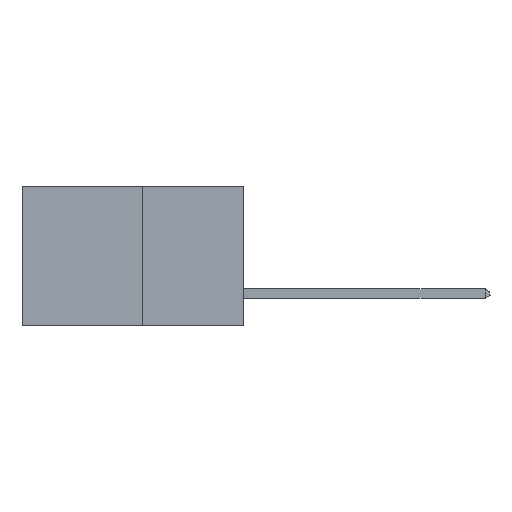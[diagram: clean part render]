
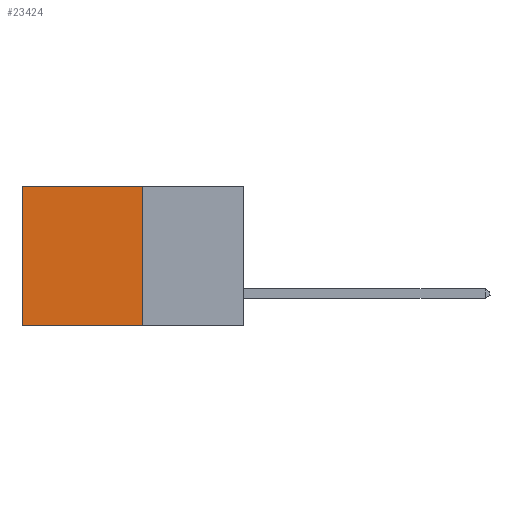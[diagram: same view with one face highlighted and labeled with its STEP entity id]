
A CAD part, left-side view. The second image highlights one B-rep face of the part: STEP entity #23424.
In plain terms, the highlighted planar face has unit normal (-1, 0, 0).
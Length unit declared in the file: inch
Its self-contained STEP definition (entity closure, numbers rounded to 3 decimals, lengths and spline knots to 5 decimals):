
#1479 = CARTESIAN_POINT ( 'NONE',  ( 0.277, 0.59, -0.37 ) ) ;
#3190 = CARTESIAN_POINT ( 'NONE',  ( 0.277, 0.27, -0.37 ) ) ;
#3373 = EDGE_LOOP ( 'NONE', ( #11371, #21034, #13658, #12511 ) ) ;
#3605 = DIRECTION ( 'NONE',  ( 0., 0., -1. ) ) ;
#3634 = CARTESIAN_POINT ( 'NONE',  ( 0.277, 0.27, -0.37 ) ) ;
#5493 = CARTESIAN_POINT ( 'NONE',  ( 0.277, 0.59, 0. ) ) ;
#5876 = AXIS2_PLACEMENT_3D ( 'NONE', #3190, #22012, #9621 ) ;
#6097 = EDGE_CURVE ( 'NONE', #18873, #8206, #9119, .T. ) ;
#6852 = FACE_OUTER_BOUND ( 'NONE', #3373, .T. ) ;
#7666 = LINE ( 'NONE', #20301, #13259 ) ;
#7858 = DIRECTION ( 'NONE',  ( 0., 1., 0. ) ) ;
#8206 = VERTEX_POINT ( 'NONE', #9523 ) ;
#9119 = LINE ( 'NONE', #3634, #24930 ) ;
#9523 = CARTESIAN_POINT ( 'NONE',  ( 0.277, 0.27, -0.37 ) ) ;
#9621 = DIRECTION ( 'NONE',  ( 0., 0., -1. ) ) ;
#10628 = CARTESIAN_POINT ( 'NONE',  ( 0.277, 0.27, -0.37 ) ) ;
#11294 = EDGE_CURVE ( 'NONE', #18873, #25038, #7666, .T. ) ;
#11371 = ORIENTED_EDGE ( 'NONE', *, *, #15181, .T. ) ;
#12090 = DIRECTION ( 'NONE',  ( 0., 0., -1. ) ) ;
#12248 = VERTEX_POINT ( 'NONE', #23499 ) ;
#12511 = ORIENTED_EDGE ( 'NONE', *, *, #11294, .T. ) ;
#13259 = VECTOR ( 'NONE', #7858, 39.37008 ) ;
#13658 = ORIENTED_EDGE ( 'NONE', *, *, #6097, .F. ) ;
#15181 = EDGE_CURVE ( 'NONE', #25038, #12248, #18478, .T. ) ;
#15876 = DIRECTION ( 'NONE',  ( 0., 1., 0. ) ) ;
#17423 = EDGE_CURVE ( 'NONE', #8206, #12248, #19270, .T. ) ;
#17828 = VECTOR ( 'NONE', #12090, 39.37008 ) ;
#18478 = LINE ( 'NONE', #1479, #17828 ) ;
#18636 = VECTOR ( 'NONE', #15876, 39.37008 ) ;
#18873 = VERTEX_POINT ( 'NONE', #20101 ) ;
#19270 = LINE ( 'NONE', #10628, #18636 ) ;
#20101 = CARTESIAN_POINT ( 'NONE',  ( 0.277, 0.27, 0. ) ) ;
#20301 = CARTESIAN_POINT ( 'NONE',  ( 0.277, 0.27, 0. ) ) ;
#21034 = ORIENTED_EDGE ( 'NONE', *, *, #17423, .F. ) ;
#21922 = PLANE ( 'NONE',  #5876 ) ;
#22012 = DIRECTION ( 'NONE',  ( 1., 0., 0. ) ) ;
#23424 = ADVANCED_FACE ( 'NONE', ( #6852 ), #21922, .F. ) ;
#23499 = CARTESIAN_POINT ( 'NONE',  ( 0.277, 0.59, -0.37 ) ) ;
#24930 = VECTOR ( 'NONE', #3605, 39.37008 ) ;
#25038 = VERTEX_POINT ( 'NONE', #5493 ) ;
